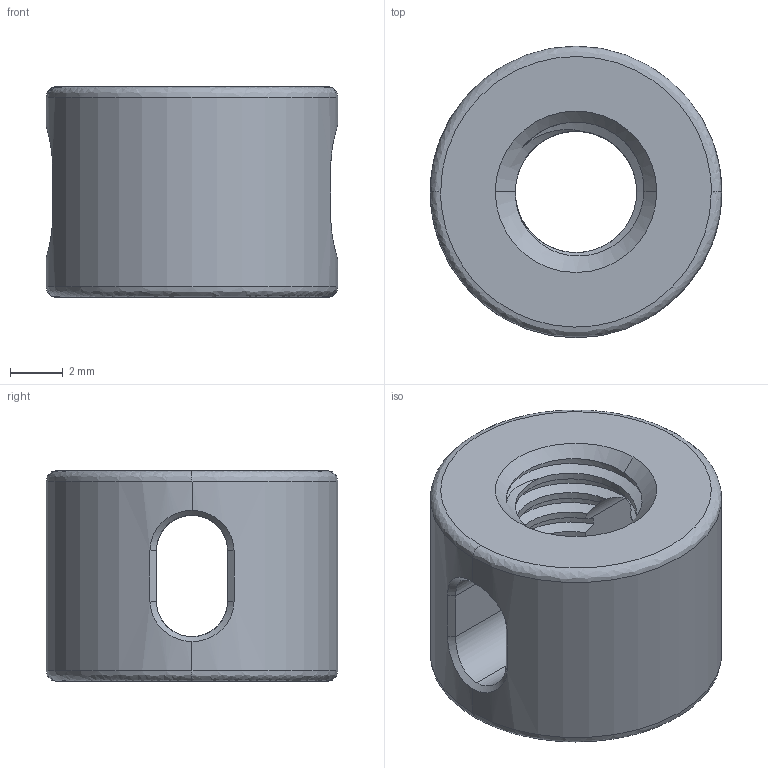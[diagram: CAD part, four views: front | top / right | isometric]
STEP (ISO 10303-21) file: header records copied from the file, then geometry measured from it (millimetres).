
FILE_DESCRIPTION (( 'STEP AP214' ), '1' );
FILE_NAME ('User Library-Telescopic Stock_Stock Bolt Nut1.STEP', '2013-05-23T12:58:05', ( 'Asher' ), ( '' ), 'SwSTEP 2.0', 'SolidWorks 2013', '' );
FILE_SCHEMA (( 'AUTOMOTIVE_DESIGN' ));
Length unit declared in the file: millimetre
Products named in the file (1): User Library-Telescopic Stock_Stock Bolt Nut1
Bounding box: 11.1 x 11.1 x 8.03 mm (x, y, z)
Volume: 542.8 mm3; surface area: 604.9 mm2
Topology: 1 solids, 1 shells, 83 faces, 242 edges, 157 vertices
Faces by surface type: cylinder 41, bspline 28, plane 10, cone 4
Entity records: 5210 total; most frequent: CARTESIAN_POINT 3457, ORIENTED_EDGE 484, EDGE_CURVE 242, DIRECTION 210, VERTEX_POINT 157, B_SPLINE_CURVE_WITH_KNOTS 92, EDGE_LOOP 85, FACE_OUTER_BOUND 83
